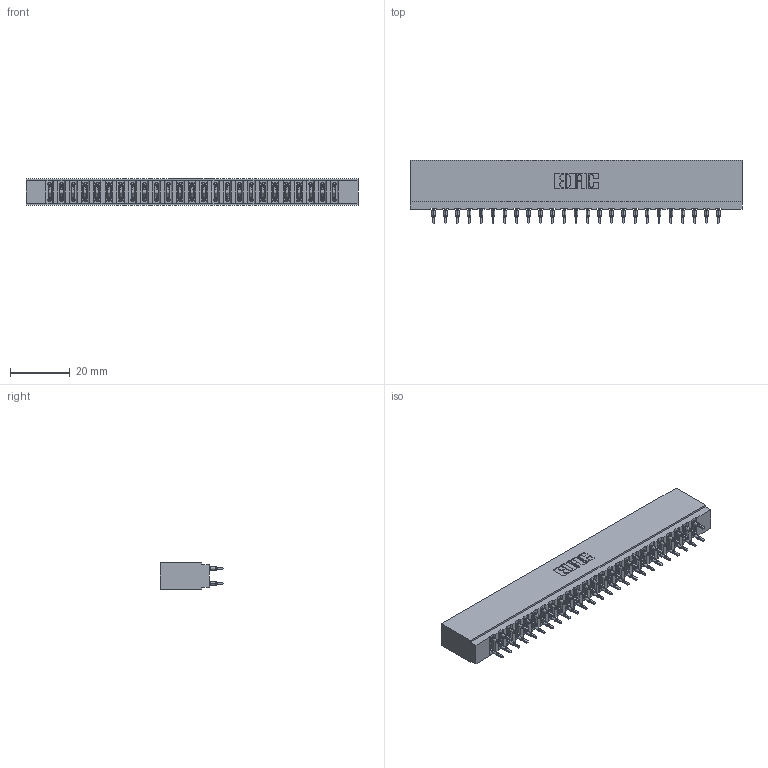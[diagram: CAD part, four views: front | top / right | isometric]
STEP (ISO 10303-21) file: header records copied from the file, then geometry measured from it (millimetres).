
FILE_DESCRIPTION (( 'STEP AP203' ), '1' );
FILE_NAME ('737-050-560-201.STEP', '2020-09-11T04:41:17', ( '' ), ( '' ), 'SwSTEP 2.0', 'SolidWorks 2020', '' );
FILE_SCHEMA (( 'CONFIG_CONTROL_DESIGN' ));
Length unit declared in the file: inch
Products named in the file (3): 737 Part_Insulator Option - 01; 745-292-001_560; 737-050-560-201
Assembly tree (51 placements, depth 2):
  737-050-560-201
    737 Part_Insulator Option - 01
    745-292-001_560  x50
Bounding box: 110.9 x 21.22 x 8.89 mm (x, y, z)
Volume: 11253.8 mm3; surface area: 16866.4 mm2
Topology: 51 solids, 51 shells, 5044 faces, 13805 edges, 8770 vertices
Faces by surface type: plane 2629, cylinder 1115, bspline 1000, torus 300
Entity records: 45530 total; most frequent: CARTESIAN_POINT 8413, ORIENTED_EDGE 7814, DIRECTION 6839, EDGE_CURVE 3907, VECTOR 3567, LINE 3567, VERTEX_POINT 2498, AXIS2_PLACEMENT_3D 1636
